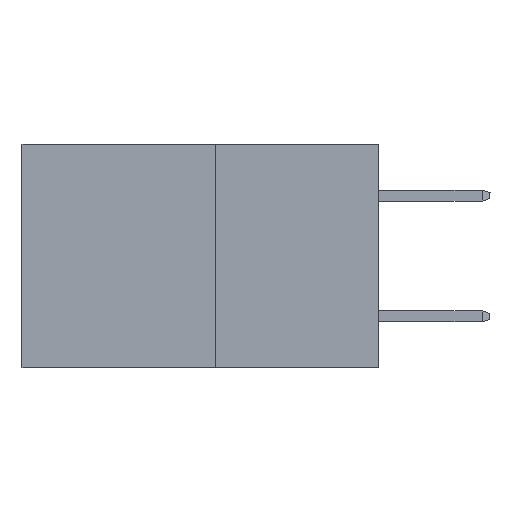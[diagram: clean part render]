
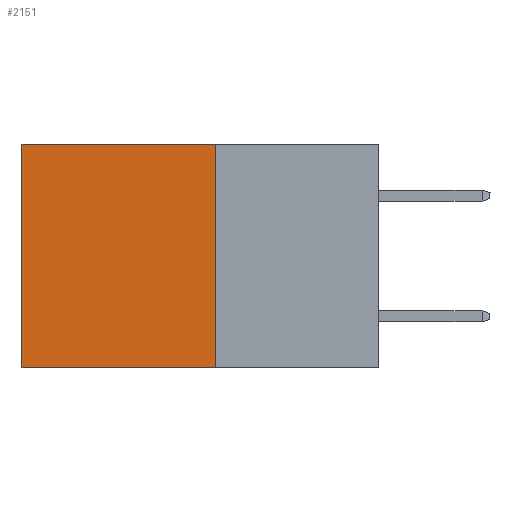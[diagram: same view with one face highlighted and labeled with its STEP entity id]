
A CAD part, left-side view. The second image highlights one B-rep face of the part: STEP entity #2151.
In plain terms, the highlighted planar face has unit normal (-1, 0, 0).
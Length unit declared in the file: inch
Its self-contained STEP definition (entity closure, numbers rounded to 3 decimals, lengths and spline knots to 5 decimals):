
#101 = DIRECTION ( 'NONE',  ( 0., 0., -1. ) ) ;
#761 = ORIENTED_EDGE ( 'NONE', *, *, #9258, .T. ) ;
#1043 = DIRECTION ( 'NONE',  ( 0., 1., 0. ) ) ;
#1258 = ORIENTED_EDGE ( 'NONE', *, *, #12921, .T. ) ;
#1411 = EDGE_CURVE ( 'NONE', #7199, #13285, #2571, .T. ) ;
#1849 = VECTOR ( 'NONE', #9702, 39.37008 ) ;
#1975 = FACE_OUTER_BOUND ( 'NONE', #9010, .T. ) ;
#2151 = ADVANCED_FACE ( 'NONE', ( #1975 ), #7248, .F. ) ;
#2304 = LINE ( 'NONE', #11483, #13774 ) ;
#2571 = LINE ( 'NONE', #3359, #8540 ) ;
#3359 = CARTESIAN_POINT ( 'NONE',  ( 0.277, 0.27, -0.37 ) ) ;
#3496 = DIRECTION ( 'NONE',  ( 0., 0., -1. ) ) ;
#4561 = CARTESIAN_POINT ( 'NONE',  ( 0.277, 0.27, -0.37 ) ) ;
#5224 = DIRECTION ( 'NONE',  ( 1., 0., 0. ) ) ;
#5530 = DIRECTION ( 'NONE',  ( 0., 1., 0. ) ) ;
#6028 = EDGE_CURVE ( 'NONE', #13285, #6980, #2304, .T. ) ;
#6510 = ORIENTED_EDGE ( 'NONE', *, *, #1411, .F. ) ;
#6557 = CARTESIAN_POINT ( 'NONE',  ( 0.277, 0.59, 0. ) ) ;
#6980 = VERTEX_POINT ( 'NONE', #8616 ) ;
#7199 = VERTEX_POINT ( 'NONE', #10182 ) ;
#7248 = PLANE ( 'NONE',  #9250 ) ;
#8195 = LINE ( 'NONE', #8227, #14779 ) ;
#8227 = CARTESIAN_POINT ( 'NONE',  ( 0.277, 0.27, 0. ) ) ;
#8499 = CARTESIAN_POINT ( 'NONE',  ( 0.277, 0.59, -0.37 ) ) ;
#8540 = VECTOR ( 'NONE', #101, 39.37008 ) ;
#8616 = CARTESIAN_POINT ( 'NONE',  ( 0.277, 0.59, -0.37 ) ) ;
#9010 = EDGE_LOOP ( 'NONE', ( #1258, #14055, #6510, #761 ) ) ;
#9250 = AXIS2_PLACEMENT_3D ( 'NONE', #11293, #5224, #3496 ) ;
#9258 = EDGE_CURVE ( 'NONE', #7199, #11914, #8195, .T. ) ;
#9702 = DIRECTION ( 'NONE',  ( 0., 0., -1. ) ) ;
#10182 = CARTESIAN_POINT ( 'NONE',  ( 0.277, 0.27, 0. ) ) ;
#11293 = CARTESIAN_POINT ( 'NONE',  ( 0.277, 0.27, -0.37 ) ) ;
#11483 = CARTESIAN_POINT ( 'NONE',  ( 0.277, 0.27, -0.37 ) ) ;
#11914 = VERTEX_POINT ( 'NONE', #6557 ) ;
#12921 = EDGE_CURVE ( 'NONE', #11914, #6980, #13696, .T. ) ;
#13285 = VERTEX_POINT ( 'NONE', #4561 ) ;
#13696 = LINE ( 'NONE', #8499, #1849 ) ;
#13774 = VECTOR ( 'NONE', #5530, 39.37008 ) ;
#14055 = ORIENTED_EDGE ( 'NONE', *, *, #6028, .F. ) ;
#14779 = VECTOR ( 'NONE', #1043, 39.37008 ) ;
